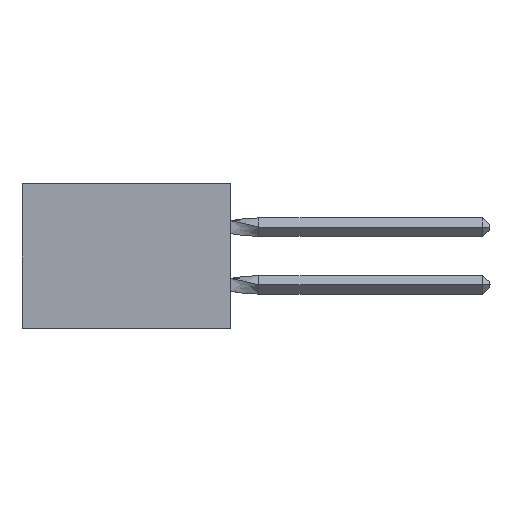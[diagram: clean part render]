
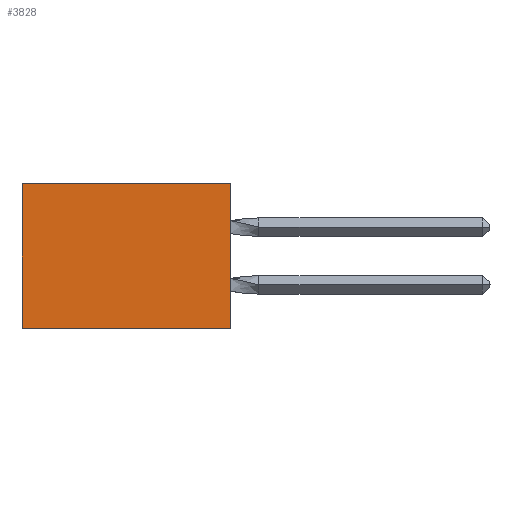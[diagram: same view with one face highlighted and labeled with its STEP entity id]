
A CAD part, left-side view. The second image highlights one B-rep face of the part: STEP entity #3828.
In plain terms, the highlighted planar face has unit normal (-1, 0, 0).
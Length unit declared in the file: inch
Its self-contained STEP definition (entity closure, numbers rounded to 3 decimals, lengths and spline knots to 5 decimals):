
#643 = AXIS2_PLACEMENT_3D ( 'NONE', #9563, #11080, #6245 ) ;
#1238 = EDGE_CURVE ( 'NONE', #18745, #14085, #1496, .T. ) ;
#1496 = LINE ( 'NONE', #7959, #16535 ) ;
#2717 = VECTOR ( 'NONE', #15109, 39.37008 ) ;
#3099 = EDGE_CURVE ( 'NONE', #12038, #18745, #8784, .T. ) ;
#3294 = FACE_OUTER_BOUND ( 'NONE', #18682, .T. ) ;
#3828 = ADVANCED_FACE ( 'NONE', ( #3294 ), #17632, .F. ) ;
#3900 = ORIENTED_EDGE ( 'NONE', *, *, #3099, .T. ) ;
#4841 = ORIENTED_EDGE ( 'NONE', *, *, #7801, .F. ) ;
#6245 = DIRECTION ( 'NONE',  ( 0., 0., -1. ) ) ;
#7008 = CARTESIAN_POINT ( 'NONE',  ( 0.305, 0., -0.5 ) ) ;
#7668 = ORIENTED_EDGE ( 'NONE', *, *, #1238, .T. ) ;
#7801 = EDGE_CURVE ( 'NONE', #12038, #9651, #15935, .T. ) ;
#7959 = CARTESIAN_POINT ( 'NONE',  ( 0.305, 0.72, -0.5 ) ) ;
#8784 = LINE ( 'NONE', #15388, #2717 ) ;
#9563 = CARTESIAN_POINT ( 'NONE',  ( 0.305, 0., -0.5 ) ) ;
#9651 = VERTEX_POINT ( 'NONE', #13359 ) ;
#10853 = VECTOR ( 'NONE', #11939, 39.37008 ) ;
#10857 = CARTESIAN_POINT ( 'NONE',  ( 0.305, 0., 0. ) ) ;
#11080 = DIRECTION ( 'NONE',  ( 1., 0., 0. ) ) ;
#11309 = ORIENTED_EDGE ( 'NONE', *, *, #15844, .F. ) ;
#11831 = CARTESIAN_POINT ( 'NONE',  ( 0.305, 0.72, -0.5 ) ) ;
#11939 = DIRECTION ( 'NONE',  ( 0., 0., -1. ) ) ;
#12038 = VERTEX_POINT ( 'NONE', #10857 ) ;
#13239 = LINE ( 'NONE', #20889, #19348 ) ;
#13359 = CARTESIAN_POINT ( 'NONE',  ( 0.305, 0., -0.5 ) ) ;
#14085 = VERTEX_POINT ( 'NONE', #11831 ) ;
#15109 = DIRECTION ( 'NONE',  ( 0., 1., 0. ) ) ;
#15388 = CARTESIAN_POINT ( 'NONE',  ( 0.305, 0., 0. ) ) ;
#15844 = EDGE_CURVE ( 'NONE', #9651, #14085, #13239, .T. ) ;
#15935 = LINE ( 'NONE', #7008, #10853 ) ;
#16535 = VECTOR ( 'NONE', #17822, 39.37008 ) ;
#17178 = DIRECTION ( 'NONE',  ( 0., 1., 0. ) ) ;
#17632 = PLANE ( 'NONE',  #643 ) ;
#17822 = DIRECTION ( 'NONE',  ( 0., 0., -1. ) ) ;
#18682 = EDGE_LOOP ( 'NONE', ( #7668, #11309, #4841, #3900 ) ) ;
#18745 = VERTEX_POINT ( 'NONE', #21044 ) ;
#19348 = VECTOR ( 'NONE', #17178, 39.37008 ) ;
#20889 = CARTESIAN_POINT ( 'NONE',  ( 0.305, 0., -0.5 ) ) ;
#21044 = CARTESIAN_POINT ( 'NONE',  ( 0.305, 0.72, 0. ) ) ;
